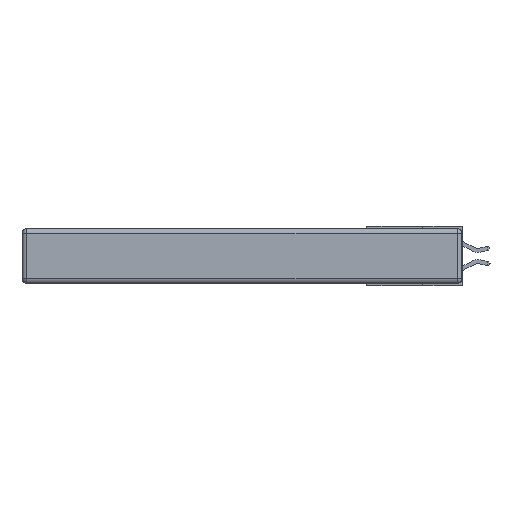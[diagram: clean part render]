
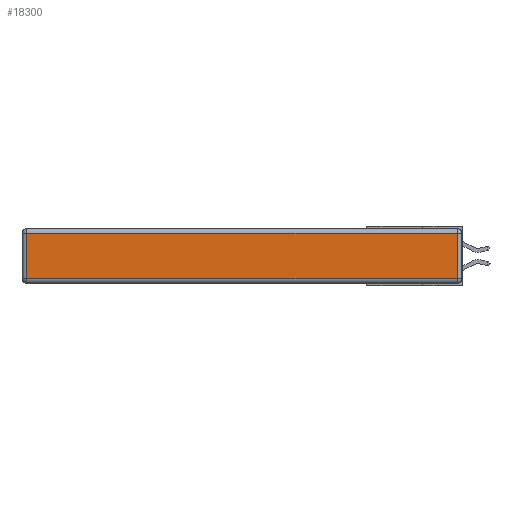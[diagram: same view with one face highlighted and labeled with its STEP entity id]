
A CAD part, left-side view. The second image highlights one B-rep face of the part: STEP entity #18300.
In plain terms, the highlighted planar face has unit normal (-1, 0, 0).
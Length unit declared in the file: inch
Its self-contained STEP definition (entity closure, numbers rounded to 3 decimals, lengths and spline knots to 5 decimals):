
#396 = LINE ( 'NONE', #10965, #18736 ) ;
#1001 = VECTOR ( 'NONE', #22541, 39.37008 ) ;
#1696 = VECTOR ( 'NONE', #12641, 39.37008 ) ;
#2307 = VERTEX_POINT ( 'NONE', #21457 ) ;
#2319 = ORIENTED_EDGE ( 'NONE', *, *, #3470, .T. ) ;
#3232 = LINE ( 'NONE', #22237, #1696 ) ;
#3353 = EDGE_CURVE ( 'NONE', #4295, #13885, #396, .T. ) ;
#3470 = EDGE_CURVE ( 'NONE', #13885, #8229, #10208, .T. ) ;
#4295 = VERTEX_POINT ( 'NONE', #9670 ) ;
#5237 = CARTESIAN_POINT ( 'NONE',  ( 0., 0., -0.313 ) ) ;
#5246 = DIRECTION ( 'NONE',  ( -1., 0., 0. ) ) ;
#7241 = DIRECTION ( 'NONE',  ( 0., 0., 1. ) ) ;
#7659 = VECTOR ( 'NONE', #23945, 39.37008 ) ;
#8229 = VERTEX_POINT ( 'NONE', #15446 ) ;
#9127 = CARTESIAN_POINT ( 'NONE',  ( 0., 0., -0.343 ) ) ;
#9670 = CARTESIAN_POINT ( 'NONE',  ( 0., 2.72, -0.03 ) ) ;
#10208 = LINE ( 'NONE', #5237, #1001 ) ;
#10965 = CARTESIAN_POINT ( 'NONE',  ( 0., 2.72, -0.343 ) ) ;
#12541 = EDGE_CURVE ( 'NONE', #8229, #2307, #12854, .T. ) ;
#12641 = DIRECTION ( 'NONE',  ( 0., 1., 0. ) ) ;
#12854 = LINE ( 'NONE', #17691, #7659 ) ;
#13885 = VERTEX_POINT ( 'NONE', #22795 ) ;
#14721 = EDGE_CURVE ( 'NONE', #2307, #4295, #3232, .T. ) ;
#14759 = ORIENTED_EDGE ( 'NONE', *, *, #3353, .T. ) ;
#15446 = CARTESIAN_POINT ( 'NONE',  ( 0., 0.03, -0.313 ) ) ;
#16226 = FACE_OUTER_BOUND ( 'NONE', #24989, .T. ) ;
#17691 = CARTESIAN_POINT ( 'NONE',  ( 0., 0.03, -0.343 ) ) ;
#18300 = ADVANCED_FACE ( 'NONE', ( #16226 ), #18837, .T. ) ;
#18736 = VECTOR ( 'NONE', #24634, 39.37008 ) ;
#18837 = PLANE ( 'NONE',  #18988 ) ;
#18988 = AXIS2_PLACEMENT_3D ( 'NONE', #9127, #5246, #7241 ) ;
#19417 = ORIENTED_EDGE ( 'NONE', *, *, #14721, .T. ) ;
#21457 = CARTESIAN_POINT ( 'NONE',  ( 0., 0.03, -0.03 ) ) ;
#22237 = CARTESIAN_POINT ( 'NONE',  ( 0., 2.75, -0.03 ) ) ;
#22538 = ORIENTED_EDGE ( 'NONE', *, *, #12541, .T. ) ;
#22541 = DIRECTION ( 'NONE',  ( 0., -1., 0. ) ) ;
#22795 = CARTESIAN_POINT ( 'NONE',  ( 0., 2.72, -0.313 ) ) ;
#23945 = DIRECTION ( 'NONE',  ( 0., 0., 1. ) ) ;
#24634 = DIRECTION ( 'NONE',  ( 0., 0., -1. ) ) ;
#24989 = EDGE_LOOP ( 'NONE', ( #2319, #22538, #19417, #14759 ) ) ;
